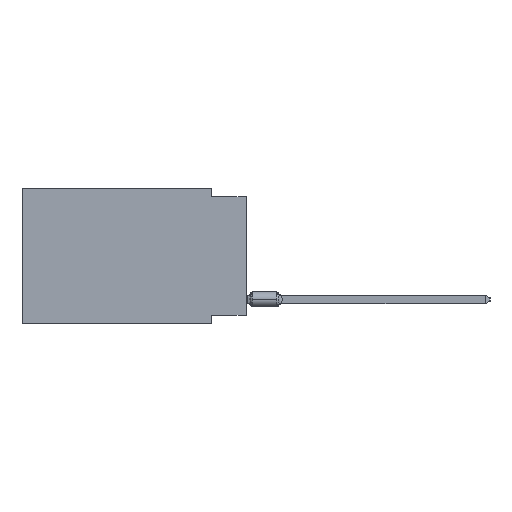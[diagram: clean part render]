
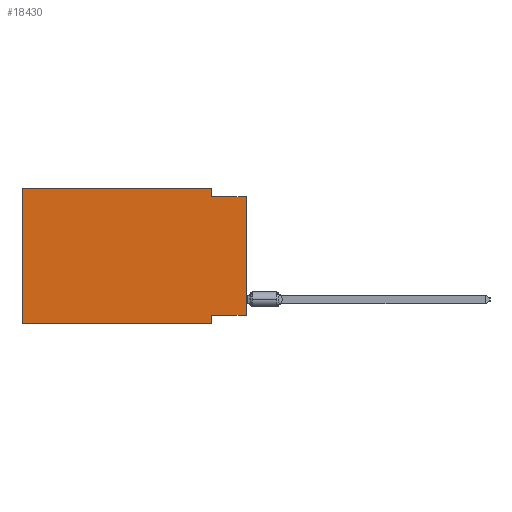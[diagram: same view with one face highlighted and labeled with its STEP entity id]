
A CAD part, left-side view. The second image highlights one B-rep face of the part: STEP entity #18430.
In plain terms, the highlighted planar face has unit normal (-1, 0, 0).
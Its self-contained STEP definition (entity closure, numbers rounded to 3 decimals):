
#2906 = CARTESIAN_POINT ( 'NONE',  ( 0., 0., 0. ) ) ;
#3308 = LINE ( 'NONE', #2906, #42444 ) ;
#4035 = DIRECTION ( 'NONE',  ( 0., -1., 0. ) ) ;
#7003 = ORIENTED_EDGE ( 'NONE', *, *, #42238, .F. ) ;
#7503 = CARTESIAN_POINT ( 'NONE',  ( 0., 16.383, 0. ) ) ;
#7873 = AXIS2_PLACEMENT_3D ( 'NONE', #48253, #23612, #30864 ) ;
#10995 = VECTOR ( 'NONE', #70425, 1000. ) ;
#13041 = LINE ( 'NONE', #73268, #25691 ) ;
#13057 = EDGE_CURVE ( 'NONE', #60138, #34578, #76438, .T. ) ;
#13859 = EDGE_LOOP ( 'NONE', ( #48865, #7003, #31123, #14539, #54812, #67864, #51275, #65344 ) ) ;
#14539 = ORIENTED_EDGE ( 'NONE', *, *, #66600, .F. ) ;
#16389 = CARTESIAN_POINT ( 'NONE',  ( 0., 2.54, 0. ) ) ;
#18430 = ADVANCED_FACE ( 'NONE', ( #23217 ), #47863, .F. ) ;
#21121 = EDGE_CURVE ( 'NONE', #52217, #67750, #62462, .T. ) ;
#21471 = CARTESIAN_POINT ( 'NONE',  ( 0., 2.54, -9.906 ) ) ;
#22889 = CARTESIAN_POINT ( 'NONE',  ( 0., 16.383, -9.906 ) ) ;
#23217 = FACE_OUTER_BOUND ( 'NONE', #13859, .T. ) ;
#23612 = DIRECTION ( 'NONE',  ( 1., 0., 0. ) ) ;
#25691 = VECTOR ( 'NONE', #74055, 1000. ) ;
#27724 = DIRECTION ( 'NONE',  ( 0., 0., -1. ) ) ;
#30864 = DIRECTION ( 'NONE',  ( 0., 0., -1. ) ) ;
#31123 = ORIENTED_EDGE ( 'NONE', *, *, #71499, .F. ) ;
#34578 = VERTEX_POINT ( 'NONE', #50199 ) ;
#34619 = DIRECTION ( 'NONE',  ( 0., -1., 0. ) ) ;
#34984 = LINE ( 'NONE', #16389, #79697 ) ;
#35666 = EDGE_CURVE ( 'NONE', #42782, #60138, #13041, .T. ) ;
#40177 = VECTOR ( 'NONE', #4035, 1000. ) ;
#40617 = CARTESIAN_POINT ( 'NONE',  ( 0., 16.383, -9.906 ) ) ;
#41879 = LINE ( 'NONE', #22889, #75664 ) ;
#42238 = EDGE_CURVE ( 'NONE', #59930, #71922, #53714, .T. ) ;
#42444 = VECTOR ( 'NONE', #46936, 1000. ) ;
#42782 = VERTEX_POINT ( 'NONE', #75282 ) ;
#42967 = VECTOR ( 'NONE', #62076, 1000. ) ;
#45780 = CARTESIAN_POINT ( 'NONE',  ( 0., 16.383, 0. ) ) ;
#46936 = DIRECTION ( 'NONE',  ( 0., 0., 1. ) ) ;
#47863 = PLANE ( 'NONE',  #7873 ) ;
#48253 = CARTESIAN_POINT ( 'NONE',  ( 0., 16.383, 0. ) ) ;
#48768 = EDGE_CURVE ( 'NONE', #52217, #34578, #41879, .T. ) ;
#48865 = ORIENTED_EDGE ( 'NONE', *, *, #73511, .T. ) ;
#50199 = CARTESIAN_POINT ( 'NONE',  ( 0., 2.54, -9.906 ) ) ;
#51275 = ORIENTED_EDGE ( 'NONE', *, *, #13057, .F. ) ;
#52217 = VERTEX_POINT ( 'NONE', #40617 ) ;
#52692 = CARTESIAN_POINT ( 'NONE',  ( 0., 0., -0.635 ) ) ;
#53714 = LINE ( 'NONE', #54915, #40177 ) ;
#54812 = ORIENTED_EDGE ( 'NONE', *, *, #21121, .F. ) ;
#54915 = CARTESIAN_POINT ( 'NONE',  ( 0., 0., -0.635 ) ) ;
#57376 = CARTESIAN_POINT ( 'NONE',  ( 0., 2.54, -9.271 ) ) ;
#57564 = CARTESIAN_POINT ( 'NONE',  ( 0., 2.54, -0.635 ) ) ;
#57914 = LINE ( 'NONE', #45780, #10995 ) ;
#58559 = CARTESIAN_POINT ( 'NONE',  ( 0., 16.383, 0. ) ) ;
#59930 = VERTEX_POINT ( 'NONE', #57564 ) ;
#60138 = VERTEX_POINT ( 'NONE', #57376 ) ;
#62076 = DIRECTION ( 'NONE',  ( 0., 0., 1. ) ) ;
#62462 = LINE ( 'NONE', #7503, #42967 ) ;
#63145 = DIRECTION ( 'NONE',  ( 0., 0., -1. ) ) ;
#65344 = ORIENTED_EDGE ( 'NONE', *, *, #35666, .F. ) ;
#66226 = VERTEX_POINT ( 'NONE', #71707 ) ;
#66600 = EDGE_CURVE ( 'NONE', #67750, #66226, #57914, .T. ) ;
#67750 = VERTEX_POINT ( 'NONE', #58559 ) ;
#67864 = ORIENTED_EDGE ( 'NONE', *, *, #48768, .T. ) ;
#70425 = DIRECTION ( 'NONE',  ( 0., -1., 0. ) ) ;
#71499 = EDGE_CURVE ( 'NONE', #66226, #59930, #34984, .T. ) ;
#71707 = CARTESIAN_POINT ( 'NONE',  ( 0., 2.54, 0. ) ) ;
#71922 = VERTEX_POINT ( 'NONE', #52692 ) ;
#73253 = VECTOR ( 'NONE', #63145, 1000. ) ;
#73268 = CARTESIAN_POINT ( 'NONE',  ( 0., 0., -9.271 ) ) ;
#73511 = EDGE_CURVE ( 'NONE', #42782, #71922, #3308, .T. ) ;
#74055 = DIRECTION ( 'NONE',  ( 0., 1., 0. ) ) ;
#75282 = CARTESIAN_POINT ( 'NONE',  ( 0., 0., -9.271 ) ) ;
#75664 = VECTOR ( 'NONE', #34619, 1000. ) ;
#76438 = LINE ( 'NONE', #21471, #73253 ) ;
#79697 = VECTOR ( 'NONE', #27724, 1000. ) ;
